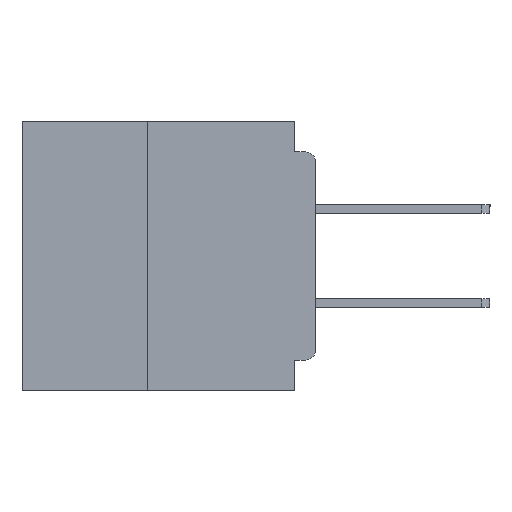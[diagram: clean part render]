
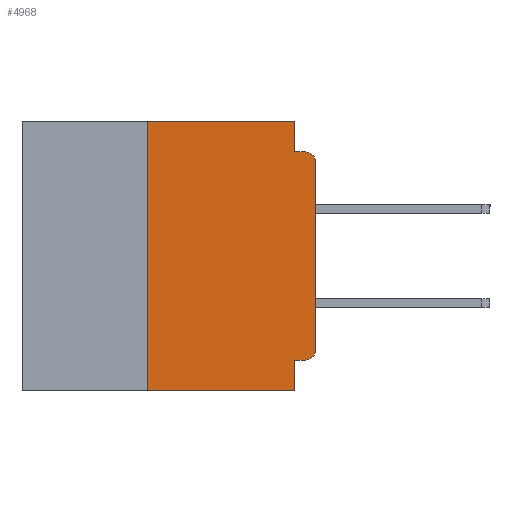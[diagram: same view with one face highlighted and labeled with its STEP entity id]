
A CAD part, left-side view. The second image highlights one B-rep face of the part: STEP entity #4968.
In plain terms, the highlighted planar face has unit normal (-1, 0, 0).
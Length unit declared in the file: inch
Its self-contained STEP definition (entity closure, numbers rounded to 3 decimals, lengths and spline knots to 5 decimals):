
#323 = DIRECTION ( 'NONE',  ( 0., 0., -1. ) ) ;
#641 = CARTESIAN_POINT ( 'NONE',  ( 0., 0.437, -0.4 ) ) ;
#1292 = CARTESIAN_POINT ( 'NONE',  ( 0., 0.25, -0.4 ) ) ;
#1457 = CARTESIAN_POINT ( 'NONE',  ( 0., 0.25, 0. ) ) ;
#2161 = VECTOR ( 'NONE', #54364, 39.37008 ) ;
#3402 = EDGE_CURVE ( 'NONE', #8739, #61178, #5081, .T. ) ;
#4968 = ADVANCED_FACE ( 'NONE', ( #27744 ), #15973, .F. ) ;
#5081 = LINE ( 'NONE', #28909, #53711 ) ;
#5411 = VECTOR ( 'NONE', #13085, 39.37008 ) ;
#5763 = CIRCLE ( 'NONE', #17193, 0.015 ) ;
#5798 = CARTESIAN_POINT ( 'NONE',  ( 0., 0.437, 0. ) ) ;
#5894 = LINE ( 'NONE', #8475, #57613 ) ;
#7395 = EDGE_CURVE ( 'NONE', #41499, #24253, #39451, .T. ) ;
#8245 = ORIENTED_EDGE ( 'NONE', *, *, #7395, .T. ) ;
#8475 = CARTESIAN_POINT ( 'NONE',  ( 0., 0., 0. ) ) ;
#8739 = VERTEX_POINT ( 'NONE', #40339 ) ;
#9081 = EDGE_CURVE ( 'NONE', #11207, #12967, #22011, .T. ) ;
#9675 = EDGE_CURVE ( 'NONE', #30897, #60224, #10851, .T. ) ;
#9917 = ORIENTED_EDGE ( 'NONE', *, *, #9081, .F. ) ;
#10851 = CIRCLE ( 'NONE', #51622, 0.015 ) ;
#11207 = VERTEX_POINT ( 'NONE', #50435 ) ;
#11402 = CARTESIAN_POINT ( 'NONE',  ( 0., 0.015, -0.34 ) ) ;
#12448 = LINE ( 'NONE', #49330, #2161 ) ;
#12748 = VECTOR ( 'NONE', #35847, 39.37008 ) ;
#12864 = CARTESIAN_POINT ( 'NONE',  ( 0., 0.031, 0. ) ) ;
#12967 = VERTEX_POINT ( 'NONE', #28866 ) ;
#13085 = DIRECTION ( 'NONE',  ( 0., 0., -1. ) ) ;
#13109 = VECTOR ( 'NONE', #323, 39.37008 ) ;
#13768 = CARTESIAN_POINT ( 'NONE',  ( 0., 0.031, -0.355 ) ) ;
#14866 = VECTOR ( 'NONE', #41582, 39.37008 ) ;
#15221 = CARTESIAN_POINT ( 'NONE',  ( 0., 0.031, -0.4 ) ) ;
#15973 = PLANE ( 'NONE',  #63872 ) ;
#16506 = DIRECTION ( 'NONE',  ( 0., 0., -1. ) ) ;
#16838 = EDGE_CURVE ( 'NONE', #8739, #55025, #5763, .T. ) ;
#17193 = AXIS2_PLACEMENT_3D ( 'NONE', #11402, #46466, #16506 ) ;
#19507 = EDGE_CURVE ( 'NONE', #41499, #58950, #56442, .T. ) ;
#21037 = DIRECTION ( 'NONE',  ( 1., 0., 0. ) ) ;
#21652 = ORIENTED_EDGE ( 'NONE', *, *, #58272, .F. ) ;
#22011 = LINE ( 'NONE', #12864, #5411 ) ;
#22362 = CARTESIAN_POINT ( 'NONE',  ( 0., 0.25, -0.4 ) ) ;
#24253 = VERTEX_POINT ( 'NONE', #15221 ) ;
#27193 = DIRECTION ( 'NONE',  ( 0., 0., 1. ) ) ;
#27744 = FACE_OUTER_BOUND ( 'NONE', #56566, .T. ) ;
#28238 = LINE ( 'NONE', #36534, #14866 ) ;
#28866 = CARTESIAN_POINT ( 'NONE',  ( 0., 0.031, -0.045 ) ) ;
#28909 = CARTESIAN_POINT ( 'NONE',  ( 0., 0., -0.355 ) ) ;
#29058 = DIRECTION ( 'NONE',  ( -1., 0., 0. ) ) ;
#30897 = VERTEX_POINT ( 'NONE', #49205 ) ;
#31462 = VECTOR ( 'NONE', #27193, 39.37008 ) ;
#35265 = ORIENTED_EDGE ( 'NONE', *, *, #16838, .T. ) ;
#35847 = DIRECTION ( 'NONE',  ( 0., -1., 0. ) ) ;
#36534 = CARTESIAN_POINT ( 'NONE',  ( 0., 0., -0.045 ) ) ;
#37164 = ORIENTED_EDGE ( 'NONE', *, *, #9675, .T. ) ;
#38712 = ORIENTED_EDGE ( 'NONE', *, *, #19507, .F. ) ;
#39451 = LINE ( 'NONE', #641, #12748 ) ;
#39812 = LINE ( 'NONE', #40379, #13109 ) ;
#40339 = CARTESIAN_POINT ( 'NONE',  ( 0., 0.015, -0.355 ) ) ;
#40379 = CARTESIAN_POINT ( 'NONE',  ( 0., 0.031, -0.4 ) ) ;
#41499 = VERTEX_POINT ( 'NONE', #1292 ) ;
#41551 = CARTESIAN_POINT ( 'NONE',  ( 0., 0., -0.34 ) ) ;
#41582 = DIRECTION ( 'NONE',  ( 0., -1., 0. ) ) ;
#43581 = DIRECTION ( 'NONE',  ( 0., 0., 1. ) ) ;
#44171 = EDGE_CURVE ( 'NONE', #55025, #30897, #5894, .T. ) ;
#44382 = ORIENTED_EDGE ( 'NONE', *, *, #64618, .F. ) ;
#46084 = CARTESIAN_POINT ( 'NONE',  ( 0., 0.015, -0.045 ) ) ;
#46466 = DIRECTION ( 'NONE',  ( -1., 0., 0. ) ) ;
#49205 = CARTESIAN_POINT ( 'NONE',  ( 0., 0., -0.06 ) ) ;
#49330 = CARTESIAN_POINT ( 'NONE',  ( 0., 0.437, 0. ) ) ;
#49904 = ORIENTED_EDGE ( 'NONE', *, *, #52844, .F. ) ;
#50435 = CARTESIAN_POINT ( 'NONE',  ( 0., 0.031, 0. ) ) ;
#51622 = AXIS2_PLACEMENT_3D ( 'NONE', #58925, #29058, #63914 ) ;
#52844 = EDGE_CURVE ( 'NONE', #58950, #11207, #12448, .T. ) ;
#53711 = VECTOR ( 'NONE', #53782, 39.37008 ) ;
#53782 = DIRECTION ( 'NONE',  ( 0., 1., 0. ) ) ;
#53798 = ORIENTED_EDGE ( 'NONE', *, *, #3402, .F. ) ;
#54364 = DIRECTION ( 'NONE',  ( 0., -1., 0. ) ) ;
#55025 = VERTEX_POINT ( 'NONE', #41551 ) ;
#55973 = DIRECTION ( 'NONE',  ( 0., 0., -1. ) ) ;
#56442 = LINE ( 'NONE', #22362, #31462 ) ;
#56566 = EDGE_LOOP ( 'NONE', ( #59157, #37164, #21652, #9917, #49904, #38712, #8245, #44382, #53798, #35265 ) ) ;
#57613 = VECTOR ( 'NONE', #43581, 39.37008 ) ;
#58272 = EDGE_CURVE ( 'NONE', #12967, #60224, #28238, .T. ) ;
#58925 = CARTESIAN_POINT ( 'NONE',  ( 0., 0.015, -0.06 ) ) ;
#58950 = VERTEX_POINT ( 'NONE', #1457 ) ;
#59157 = ORIENTED_EDGE ( 'NONE', *, *, #44171, .T. ) ;
#60224 = VERTEX_POINT ( 'NONE', #46084 ) ;
#61178 = VERTEX_POINT ( 'NONE', #13768 ) ;
#63872 = AXIS2_PLACEMENT_3D ( 'NONE', #5798, #21037, #55973 ) ;
#63914 = DIRECTION ( 'NONE',  ( 0., 0., -1. ) ) ;
#64618 = EDGE_CURVE ( 'NONE', #61178, #24253, #39812, .T. ) ;
